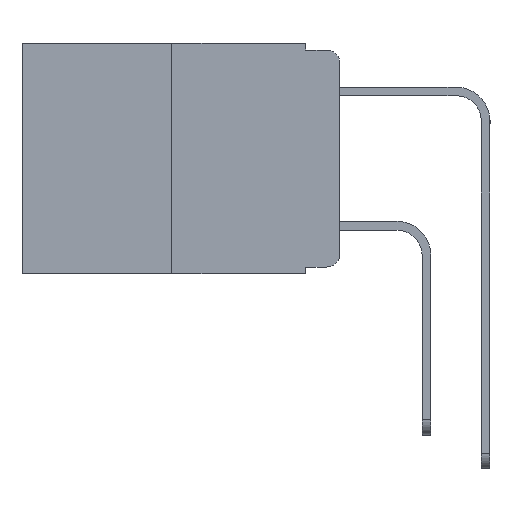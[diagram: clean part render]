
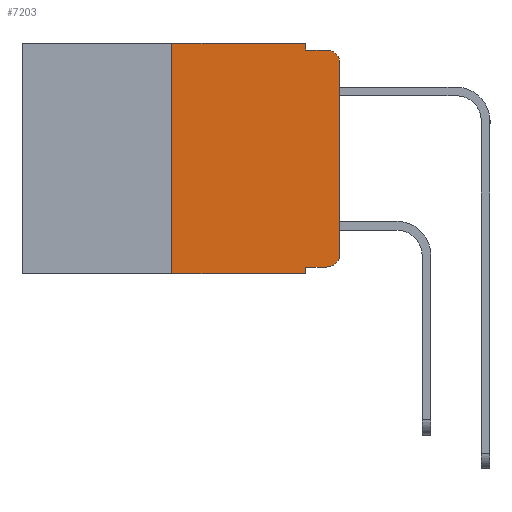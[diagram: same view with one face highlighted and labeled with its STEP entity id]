
A CAD part, left-side view. The second image highlights one B-rep face of the part: STEP entity #7203.
In plain terms, the highlighted planar face has unit normal (-1, 0, 0).
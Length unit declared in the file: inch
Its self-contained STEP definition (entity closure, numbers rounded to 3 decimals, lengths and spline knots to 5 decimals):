
#49 = VERTEX_POINT ( 'NONE', #12105 ) ;
#61 = LINE ( 'NONE', #3268, #8510 ) ;
#984 = EDGE_LOOP ( 'NONE', ( #11738, #7769, #4237, #8427, #2695, #4412, #4072, #3554, #5097, #7457 ) ) ;
#1913 = VECTOR ( 'NONE', #12119, 39.37008 ) ;
#1929 = DIRECTION ( 'NONE',  ( 0., 0., -1. ) ) ;
#2131 = DIRECTION ( 'NONE',  ( -1., 0., 0. ) ) ;
#2404 = CARTESIAN_POINT ( 'NONE',  ( 0., 0.25, 0. ) ) ;
#2588 = CARTESIAN_POINT ( 'NONE',  ( 0., 0.051, 0. ) ) ;
#2695 = ORIENTED_EDGE ( 'NONE', *, *, #6275, .F. ) ;
#2700 = VERTEX_POINT ( 'NONE', #10990 ) ;
#2752 = AXIS2_PLACEMENT_3D ( 'NONE', #9825, #9762, #9781 ) ;
#2849 = VECTOR ( 'NONE', #12075, 39.37008 ) ;
#3111 = CIRCLE ( 'NONE', #3563, 0.02 ) ;
#3174 = VERTEX_POINT ( 'NONE', #6229 ) ;
#3258 = DIRECTION ( 'NONE',  ( 0., -1., 0. ) ) ;
#3268 = CARTESIAN_POINT ( 'NONE',  ( 0., 0.473, 0. ) ) ;
#3554 = ORIENTED_EDGE ( 'NONE', *, *, #3835, .F. ) ;
#3563 = AXIS2_PLACEMENT_3D ( 'NONE', #5704, #5691, #9399 ) ;
#3828 = CARTESIAN_POINT ( 'NONE',  ( 0., 0., 0. ) ) ;
#3835 = EDGE_CURVE ( 'NONE', #3174, #4677, #7704, .T. ) ;
#4072 = ORIENTED_EDGE ( 'NONE', *, *, #9799, .T. ) ;
#4117 = EDGE_CURVE ( 'NONE', #7496, #5799, #5736, .T. ) ;
#4237 = ORIENTED_EDGE ( 'NONE', *, *, #5490, .F. ) ;
#4411 = VECTOR ( 'NONE', #12902, 39.37008 ) ;
#4412 = ORIENTED_EDGE ( 'NONE', *, *, #11923, .F. ) ;
#4525 = LINE ( 'NONE', #4713, #9890 ) ;
#4677 = VERTEX_POINT ( 'NONE', #12923 ) ;
#4713 = CARTESIAN_POINT ( 'NONE',  ( 0., 0.051, -0.333 ) ) ;
#4807 = CIRCLE ( 'NONE', #12377, 0.02 ) ;
#4852 = EDGE_CURVE ( 'NONE', #49, #2700, #10568, .T. ) ;
#4899 = VECTOR ( 'NONE', #1929, 39.37008 ) ;
#4952 = VERTEX_POINT ( 'NONE', #6911 ) ;
#5043 = VECTOR ( 'NONE', #5044, 39.37008 ) ;
#5044 = DIRECTION ( 'NONE',  ( 0., -1., 0. ) ) ;
#5097 = ORIENTED_EDGE ( 'NONE', *, *, #5738, .T. ) ;
#5204 = CARTESIAN_POINT ( 'NONE',  ( 0., 0., -0.03 ) ) ;
#5349 = VERTEX_POINT ( 'NONE', #6099 ) ;
#5486 = VECTOR ( 'NONE', #9944, 39.37008 ) ;
#5490 = EDGE_CURVE ( 'NONE', #2700, #8971, #13437, .T. ) ;
#5519 = CARTESIAN_POINT ( 'NONE',  ( 0., 0.473, -0.343 ) ) ;
#5691 = DIRECTION ( 'NONE',  ( -1., 0., 0. ) ) ;
#5704 = CARTESIAN_POINT ( 'NONE',  ( 0., 0.02, -0.03 ) ) ;
#5736 = LINE ( 'NONE', #3828, #2849 ) ;
#5738 = EDGE_CURVE ( 'NONE', #3174, #4952, #4525, .T. ) ;
#5799 = VERTEX_POINT ( 'NONE', #5204 ) ;
#5874 = CARTESIAN_POINT ( 'NONE',  ( 0., 0.051, 0. ) ) ;
#6099 = CARTESIAN_POINT ( 'NONE',  ( 0., 0.25, 0. ) ) ;
#6229 = CARTESIAN_POINT ( 'NONE',  ( 0., 0.051, -0.333 ) ) ;
#6274 = EDGE_CURVE ( 'NONE', #5799, #8971, #3111, .T. ) ;
#6275 = EDGE_CURVE ( 'NONE', #5349, #49, #61, .T. ) ;
#6911 = CARTESIAN_POINT ( 'NONE',  ( 0., 0.02, -0.333 ) ) ;
#7087 = CARTESIAN_POINT ( 'NONE',  ( 0., 0.02, -0.01 ) ) ;
#7203 = ADVANCED_FACE ( 'NONE', ( #8007 ), #10881, .F. ) ;
#7234 = VERTEX_POINT ( 'NONE', #13392 ) ;
#7271 = LINE ( 'NONE', #5519, #4411 ) ;
#7457 = ORIENTED_EDGE ( 'NONE', *, *, #12412, .T. ) ;
#7496 = VERTEX_POINT ( 'NONE', #13347 ) ;
#7704 = LINE ( 'NONE', #5874, #1913 ) ;
#7769 = ORIENTED_EDGE ( 'NONE', *, *, #6274, .T. ) ;
#8007 = FACE_OUTER_BOUND ( 'NONE', #984, .T. ) ;
#8427 = ORIENTED_EDGE ( 'NONE', *, *, #4852, .F. ) ;
#8481 = DIRECTION ( 'NONE',  ( 0., -1., 0. ) ) ;
#8510 = VECTOR ( 'NONE', #3258, 39.37008 ) ;
#8608 = CARTESIAN_POINT ( 'NONE',  ( 0., 0.02, -0.313 ) ) ;
#8971 = VERTEX_POINT ( 'NONE', #7087 ) ;
#9203 = CARTESIAN_POINT ( 'NONE',  ( 0., 0.051, -0.01 ) ) ;
#9399 = DIRECTION ( 'NONE',  ( 0., 0., -1. ) ) ;
#9698 = DIRECTION ( 'NONE',  ( 0., 0., -1. ) ) ;
#9762 = DIRECTION ( 'NONE',  ( 1., 0., 0. ) ) ;
#9781 = DIRECTION ( 'NONE',  ( 0., 0., -1. ) ) ;
#9799 = EDGE_CURVE ( 'NONE', #7234, #4677, #7271, .T. ) ;
#9825 = CARTESIAN_POINT ( 'NONE',  ( 0., 0.473, 0. ) ) ;
#9890 = VECTOR ( 'NONE', #8481, 39.37008 ) ;
#9944 = DIRECTION ( 'NONE',  ( 0., 0., 1. ) ) ;
#10568 = LINE ( 'NONE', #2588, #4899 ) ;
#10825 = LINE ( 'NONE', #2404, #5486 ) ;
#10881 = PLANE ( 'NONE',  #2752 ) ;
#10990 = CARTESIAN_POINT ( 'NONE',  ( 0., 0.051, -0.01 ) ) ;
#11738 = ORIENTED_EDGE ( 'NONE', *, *, #4117, .T. ) ;
#11923 = EDGE_CURVE ( 'NONE', #7234, #5349, #10825, .T. ) ;
#12075 = DIRECTION ( 'NONE',  ( 0., 0., 1. ) ) ;
#12105 = CARTESIAN_POINT ( 'NONE',  ( 0., 0.051, 0. ) ) ;
#12119 = DIRECTION ( 'NONE',  ( 0., 0., -1. ) ) ;
#12377 = AXIS2_PLACEMENT_3D ( 'NONE', #8608, #2131, #9698 ) ;
#12412 = EDGE_CURVE ( 'NONE', #4952, #7496, #4807, .T. ) ;
#12902 = DIRECTION ( 'NONE',  ( 0., -1., 0. ) ) ;
#12923 = CARTESIAN_POINT ( 'NONE',  ( 0., 0.051, -0.343 ) ) ;
#13347 = CARTESIAN_POINT ( 'NONE',  ( 0., 0., -0.313 ) ) ;
#13392 = CARTESIAN_POINT ( 'NONE',  ( 0., 0.25, -0.343 ) ) ;
#13437 = LINE ( 'NONE', #9203, #5043 ) ;
